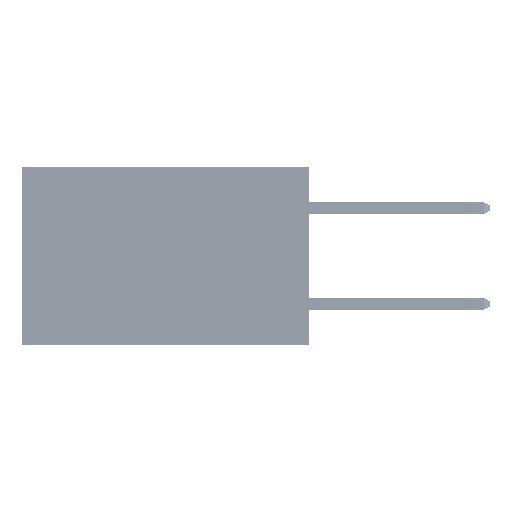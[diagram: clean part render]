
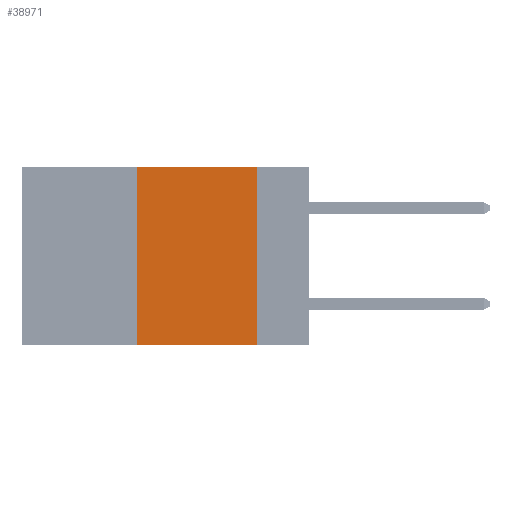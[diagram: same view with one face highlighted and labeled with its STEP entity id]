
A CAD part, left-side view. The second image highlights one B-rep face of the part: STEP entity #38971.
In plain terms, the highlighted planar face has unit normal (-1, 0, 0).
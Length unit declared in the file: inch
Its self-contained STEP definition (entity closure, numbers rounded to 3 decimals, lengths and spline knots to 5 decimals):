
#1279 = ORIENTED_EDGE ( 'NONE', *, *, #7078, .F. ) ;
#2111 = LINE ( 'NONE', #22809, #22598 ) ;
#7078 = EDGE_CURVE ( 'NONE', #45198, #11912, #36687, .T. ) ;
#9214 = LINE ( 'NONE', #38982, #24647 ) ;
#10784 = VERTEX_POINT ( 'NONE', #21961 ) ;
#11912 = VERTEX_POINT ( 'NONE', #44489 ) ;
#12761 = PLANE ( 'NONE',  #19277 ) ;
#15031 = CARTESIAN_POINT ( 'NONE',  ( 0., 0.11, -0.37 ) ) ;
#17035 = EDGE_CURVE ( 'NONE', #11912, #21286, #2111, .T. ) ;
#18528 = DIRECTION ( 'NONE',  ( 0., 0., -1. ) ) ;
#19277 = AXIS2_PLACEMENT_3D ( 'NONE', #33941, #21635, #28603 ) ;
#19988 = CARTESIAN_POINT ( 'NONE',  ( 0., 0.36, 0. ) ) ;
#20916 = EDGE_LOOP ( 'NONE', ( #45182, #1279, #27197, #52853 ) ) ;
#21286 = VERTEX_POINT ( 'NONE', #15031 ) ;
#21635 = DIRECTION ( 'NONE',  ( 1., 0., 0. ) ) ;
#21961 = CARTESIAN_POINT ( 'NONE',  ( 0., 0.36, -0.37 ) ) ;
#22598 = VECTOR ( 'NONE', #18528, 39.37008 ) ;
#22809 = CARTESIAN_POINT ( 'NONE',  ( 0., 0.11, 0. ) ) ;
#23453 = LINE ( 'NONE', #19988, #41751 ) ;
#24647 = VECTOR ( 'NONE', #30414, 39.37008 ) ;
#27197 = ORIENTED_EDGE ( 'NONE', *, *, #43851, .F. ) ;
#28284 = CARTESIAN_POINT ( 'NONE',  ( 0., 0.36, 0. ) ) ;
#28603 = DIRECTION ( 'NONE',  ( 0., 0., -1. ) ) ;
#30414 = DIRECTION ( 'NONE',  ( 0., -1., 0. ) ) ;
#33941 = CARTESIAN_POINT ( 'NONE',  ( 0., 0.6, 0. ) ) ;
#36687 = LINE ( 'NONE', #42046, #52269 ) ;
#38971 = ADVANCED_FACE ( 'NONE', ( #42013 ), #12761, .F. ) ;
#38982 = CARTESIAN_POINT ( 'NONE',  ( 0., 0.6, -0.37 ) ) ;
#41751 = VECTOR ( 'NONE', #48419, 39.37008 ) ;
#42013 = FACE_OUTER_BOUND ( 'NONE', #20916, .T. ) ;
#42046 = CARTESIAN_POINT ( 'NONE',  ( 0., 0.6, 0. ) ) ;
#43851 = EDGE_CURVE ( 'NONE', #10784, #45198, #23453, .T. ) ;
#44489 = CARTESIAN_POINT ( 'NONE',  ( 0., 0.11, 0. ) ) ;
#45182 = ORIENTED_EDGE ( 'NONE', *, *, #17035, .F. ) ;
#45198 = VERTEX_POINT ( 'NONE', #28284 ) ;
#45429 = DIRECTION ( 'NONE',  ( 0., -1., 0. ) ) ;
#48419 = DIRECTION ( 'NONE',  ( 0., 0., 1. ) ) ;
#50346 = EDGE_CURVE ( 'NONE', #10784, #21286, #9214, .T. ) ;
#52269 = VECTOR ( 'NONE', #45429, 39.37008 ) ;
#52853 = ORIENTED_EDGE ( 'NONE', *, *, #50346, .T. ) ;
